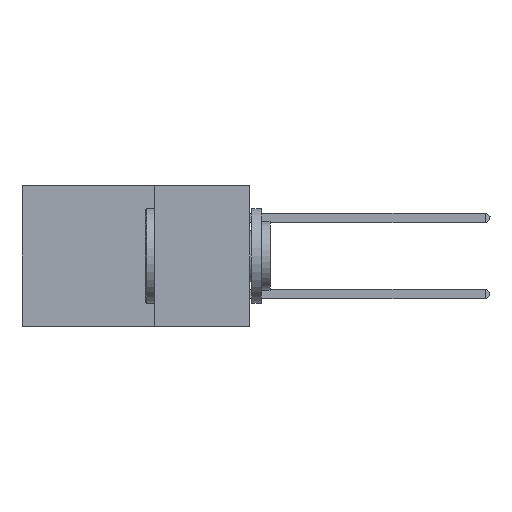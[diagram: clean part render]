
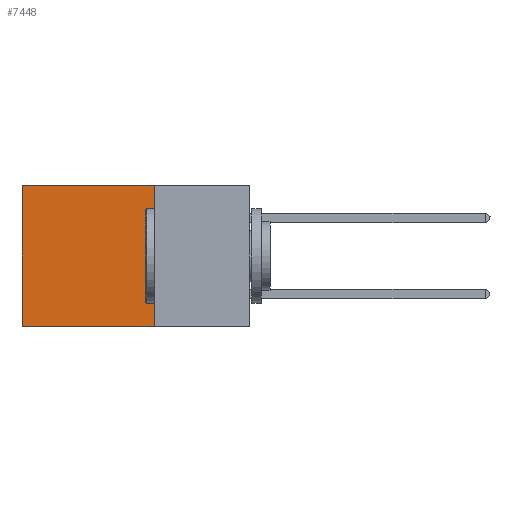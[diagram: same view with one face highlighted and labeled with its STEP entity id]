
A CAD part, left-side view. The second image highlights one B-rep face of the part: STEP entity #7448.
In plain terms, the highlighted planar face has unit normal (-1, 0, 0).
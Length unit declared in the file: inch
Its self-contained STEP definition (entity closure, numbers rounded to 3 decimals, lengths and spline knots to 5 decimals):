
#260 = EDGE_CURVE ( 'NONE', #12604, #8739, #491, .T. ) ;
#264 = LINE ( 'NONE', #5804, #3207 ) ;
#491 = LINE ( 'NONE', #15422, #11123 ) ;
#985 = DIRECTION ( 'NONE',  ( 0., 1., 0. ) ) ;
#1139 = PLANE ( 'NONE',  #16831 ) ;
#2422 = CARTESIAN_POINT ( 'NONE',  ( 0.2875, 0.6, 0. ) ) ;
#3181 = LINE ( 'NONE', #15166, #18090 ) ;
#3207 = VECTOR ( 'NONE', #985, 39.37008 ) ;
#4063 = CARTESIAN_POINT ( 'NONE',  ( 0.2875, 0.25, 0. ) ) ;
#4982 = DIRECTION ( 'NONE',  ( 0., 0., -1. ) ) ;
#5804 = CARTESIAN_POINT ( 'NONE',  ( 0.2875, 0.25, -0.37 ) ) ;
#5872 = ORIENTED_EDGE ( 'NONE', *, *, #18613, .F. ) ;
#5877 = VECTOR ( 'NONE', #4982, 39.37008 ) ;
#6446 = CARTESIAN_POINT ( 'NONE',  ( 0.2875, 0.25, -0.37 ) ) ;
#6544 = EDGE_CURVE ( 'NONE', #12604, #13958, #3181, .T. ) ;
#6922 = EDGE_CURVE ( 'NONE', #8739, #11041, #10830, .T. ) ;
#7308 = ORIENTED_EDGE ( 'NONE', *, *, #260, .T. ) ;
#7402 = DIRECTION ( 'NONE',  ( 0., 0., -1. ) ) ;
#7448 = ADVANCED_FACE ( 'NONE', ( #8358 ), #1139, .F. ) ;
#8358 = FACE_OUTER_BOUND ( 'NONE', #11740, .T. ) ;
#8739 = VERTEX_POINT ( 'NONE', #2422 ) ;
#9248 = CARTESIAN_POINT ( 'NONE',  ( 0.2875, 0.6, 0. ) ) ;
#9389 = DIRECTION ( 'NONE',  ( 1., 0., 0. ) ) ;
#9528 = CARTESIAN_POINT ( 'NONE',  ( 0.2875, 0.6, -0.37 ) ) ;
#10747 = DIRECTION ( 'NONE',  ( 0., 0., -1. ) ) ;
#10830 = LINE ( 'NONE', #9248, #5877 ) ;
#11041 = VERTEX_POINT ( 'NONE', #9528 ) ;
#11069 = ORIENTED_EDGE ( 'NONE', *, *, #6544, .F. ) ;
#11123 = VECTOR ( 'NONE', #18458, 39.37008 ) ;
#11253 = ORIENTED_EDGE ( 'NONE', *, *, #6922, .T. ) ;
#11740 = EDGE_LOOP ( 'NONE', ( #11253, #5872, #11069, #7308 ) ) ;
#12604 = VERTEX_POINT ( 'NONE', #14989 ) ;
#13958 = VERTEX_POINT ( 'NONE', #6446 ) ;
#14989 = CARTESIAN_POINT ( 'NONE',  ( 0.2875, 0.25, 0. ) ) ;
#15166 = CARTESIAN_POINT ( 'NONE',  ( 0.2875, 0.25, 0. ) ) ;
#15422 = CARTESIAN_POINT ( 'NONE',  ( 0.2875, 0.25, 0. ) ) ;
#16831 = AXIS2_PLACEMENT_3D ( 'NONE', #4063, #9389, #7402 ) ;
#18090 = VECTOR ( 'NONE', #10747, 39.37008 ) ;
#18458 = DIRECTION ( 'NONE',  ( 0., 1., 0. ) ) ;
#18613 = EDGE_CURVE ( 'NONE', #13958, #11041, #264, .T. ) ;
